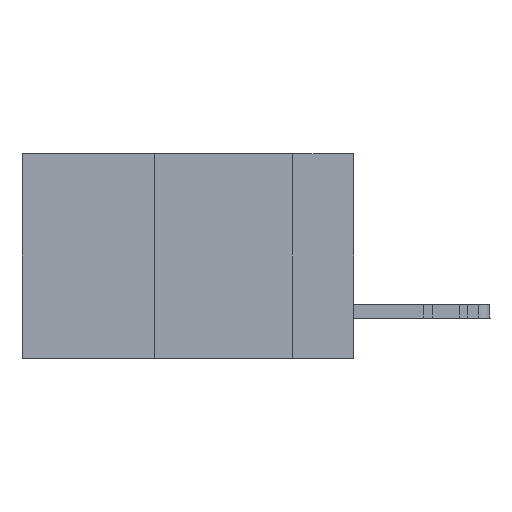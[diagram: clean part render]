
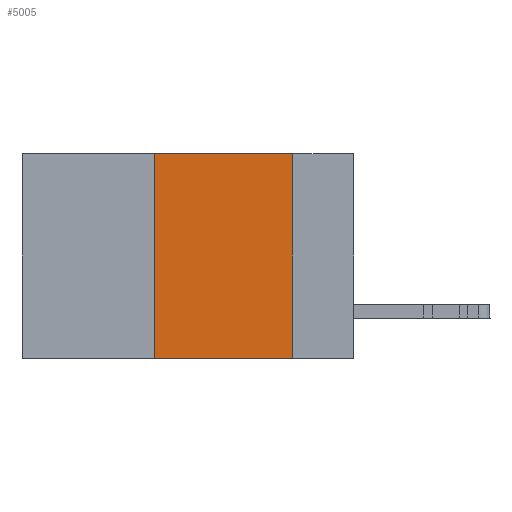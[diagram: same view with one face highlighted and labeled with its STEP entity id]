
A CAD part, left-side view. The second image highlights one B-rep face of the part: STEP entity #5005.
In plain terms, the highlighted planar face has unit normal (-1, 0, 0).
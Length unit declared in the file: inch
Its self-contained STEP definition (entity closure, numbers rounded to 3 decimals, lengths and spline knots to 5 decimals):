
#2104 = CARTESIAN_POINT ( 'NONE',  ( 0., 0.36, -0.37 ) ) ;
#2689 = EDGE_CURVE ( 'NONE', #6849, #44966, #28845, .T. ) ;
#2731 = EDGE_LOOP ( 'NONE', ( #46508, #33782, #28661, #31613 ) ) ;
#4509 = DIRECTION ( 'NONE',  ( 0., -1., 0. ) ) ;
#5005 = ADVANCED_FACE ( 'NONE', ( #7961 ), #9192, .F. ) ;
#5632 = CARTESIAN_POINT ( 'NONE',  ( 0., 0.6, 0. ) ) ;
#6849 = VERTEX_POINT ( 'NONE', #32186 ) ;
#7883 = VERTEX_POINT ( 'NONE', #16137 ) ;
#7961 = FACE_OUTER_BOUND ( 'NONE', #2731, .T. ) ;
#9192 = PLANE ( 'NONE',  #38935 ) ;
#14091 = DIRECTION ( 'NONE',  ( 0., 0., -1. ) ) ;
#14884 = VERTEX_POINT ( 'NONE', #2104 ) ;
#16012 = EDGE_CURVE ( 'NONE', #14884, #7883, #35319, .T. ) ;
#16137 = CARTESIAN_POINT ( 'NONE',  ( 0., 0.36, 0. ) ) ;
#18084 = CARTESIAN_POINT ( 'NONE',  ( 0., 0.6, 0. ) ) ;
#20030 = DIRECTION ( 'NONE',  ( 1., 0., 0. ) ) ;
#21118 = CARTESIAN_POINT ( 'NONE',  ( 0., 0.11, 0. ) ) ;
#21351 = CARTESIAN_POINT ( 'NONE',  ( 0., 0.11, -0.37 ) ) ;
#22175 = CARTESIAN_POINT ( 'NONE',  ( 0., 0.36, 0. ) ) ;
#24346 = LINE ( 'NONE', #18084, #32994 ) ;
#24391 = DIRECTION ( 'NONE',  ( 0., 0., -1. ) ) ;
#26035 = EDGE_CURVE ( 'NONE', #7883, #6849, #24346, .T. ) ;
#28661 = ORIENTED_EDGE ( 'NONE', *, *, #16012, .F. ) ;
#28845 = LINE ( 'NONE', #21118, #40330 ) ;
#31613 = ORIENTED_EDGE ( 'NONE', *, *, #40584, .T. ) ;
#32186 = CARTESIAN_POINT ( 'NONE',  ( 0., 0.11, 0. ) ) ;
#32302 = DIRECTION ( 'NONE',  ( 0., -1., 0. ) ) ;
#32308 = VECTOR ( 'NONE', #4509, 39.37008 ) ;
#32994 = VECTOR ( 'NONE', #32302, 39.37008 ) ;
#33782 = ORIENTED_EDGE ( 'NONE', *, *, #26035, .F. ) ;
#34764 = VECTOR ( 'NONE', #43967, 39.37008 ) ;
#35319 = LINE ( 'NONE', #22175, #34764 ) ;
#38935 = AXIS2_PLACEMENT_3D ( 'NONE', #5632, #20030, #24391 ) ;
#40330 = VECTOR ( 'NONE', #14091, 39.37008 ) ;
#40584 = EDGE_CURVE ( 'NONE', #14884, #44966, #42651, .T. ) ;
#42651 = LINE ( 'NONE', #45038, #32308 ) ;
#43967 = DIRECTION ( 'NONE',  ( 0., 0., 1. ) ) ;
#44966 = VERTEX_POINT ( 'NONE', #21351 ) ;
#45038 = CARTESIAN_POINT ( 'NONE',  ( 0., 0.6, -0.37 ) ) ;
#46508 = ORIENTED_EDGE ( 'NONE', *, *, #2689, .F. ) ;
